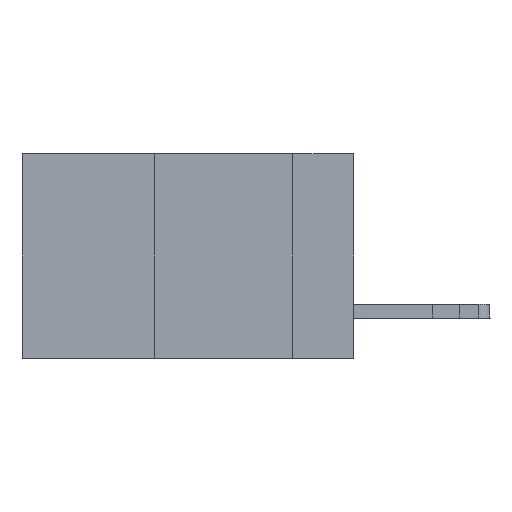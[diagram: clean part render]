
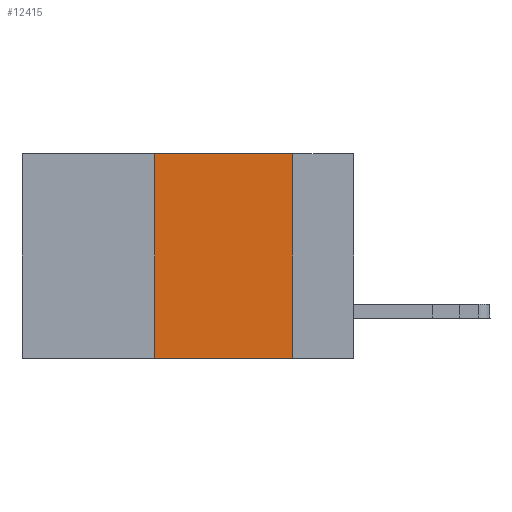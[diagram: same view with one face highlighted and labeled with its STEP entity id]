
A CAD part, left-side view. The second image highlights one B-rep face of the part: STEP entity #12415.
In plain terms, the highlighted planar face has unit normal (-1, 0, 0).
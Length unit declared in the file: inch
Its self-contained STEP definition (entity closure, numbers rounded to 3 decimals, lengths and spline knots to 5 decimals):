
#502 = CARTESIAN_POINT ( 'NONE',  ( 0., 0.11, 0. ) ) ;
#864 = VERTEX_POINT ( 'NONE', #7606 ) ;
#1895 = DIRECTION ( 'NONE',  ( 0., 0., 1. ) ) ;
#1933 = LINE ( 'NONE', #12898, #21300 ) ;
#2849 = ORIENTED_EDGE ( 'NONE', *, *, #12325, .F. ) ;
#4707 = VECTOR ( 'NONE', #1895, 39.37008 ) ;
#6013 = VERTEX_POINT ( 'NONE', #8427 ) ;
#6501 = CARTESIAN_POINT ( 'NONE',  ( 0., 0.36, 0. ) ) ;
#6968 = EDGE_LOOP ( 'NONE', ( #19712, #2849, #7848, #15375 ) ) ;
#7606 = CARTESIAN_POINT ( 'NONE',  ( 0., 0.36, -0.37 ) ) ;
#7848 = ORIENTED_EDGE ( 'NONE', *, *, #14499, .F. ) ;
#8414 = LINE ( 'NONE', #14789, #4707 ) ;
#8427 = CARTESIAN_POINT ( 'NONE',  ( 0., 0.11, 0. ) ) ;
#8536 = LINE ( 'NONE', #502, #22427 ) ;
#10918 = DIRECTION ( 'NONE',  ( 1., 0., 0. ) ) ;
#12325 = EDGE_CURVE ( 'NONE', #18963, #6013, #19388, .T. ) ;
#12415 = ADVANCED_FACE ( 'NONE', ( #18269 ), #21726, .F. ) ;
#12470 = EDGE_CURVE ( 'NONE', #864, #22399, #1933, .T. ) ;
#12898 = CARTESIAN_POINT ( 'NONE',  ( 0., 0.6, -0.37 ) ) ;
#14499 = EDGE_CURVE ( 'NONE', #864, #18963, #8414, .T. ) ;
#14726 = DIRECTION ( 'NONE',  ( 0., -1., 0. ) ) ;
#14789 = CARTESIAN_POINT ( 'NONE',  ( 0., 0.36, 0. ) ) ;
#15375 = ORIENTED_EDGE ( 'NONE', *, *, #12470, .T. ) ;
#16113 = CARTESIAN_POINT ( 'NONE',  ( 0., 0.11, -0.37 ) ) ;
#16371 = CARTESIAN_POINT ( 'NONE',  ( 0., 0.6, 0. ) ) ;
#17069 = DIRECTION ( 'NONE',  ( 0., 0., -1. ) ) ;
#17834 = CARTESIAN_POINT ( 'NONE',  ( 0., 0.6, 0. ) ) ;
#18269 = FACE_OUTER_BOUND ( 'NONE', #6968, .T. ) ;
#18963 = VERTEX_POINT ( 'NONE', #6501 ) ;
#19388 = LINE ( 'NONE', #17834, #23518 ) ;
#19712 = ORIENTED_EDGE ( 'NONE', *, *, #23299, .F. ) ;
#21300 = VECTOR ( 'NONE', #14726, 39.37008 ) ;
#21408 = DIRECTION ( 'NONE',  ( 0., -1., 0. ) ) ;
#21726 = PLANE ( 'NONE',  #22134 ) ;
#22134 = AXIS2_PLACEMENT_3D ( 'NONE', #16371, #10918, #23488 ) ;
#22399 = VERTEX_POINT ( 'NONE', #16113 ) ;
#22427 = VECTOR ( 'NONE', #17069, 39.37008 ) ;
#23299 = EDGE_CURVE ( 'NONE', #6013, #22399, #8536, .T. ) ;
#23488 = DIRECTION ( 'NONE',  ( 0., 0., -1. ) ) ;
#23518 = VECTOR ( 'NONE', #21408, 39.37008 ) ;
